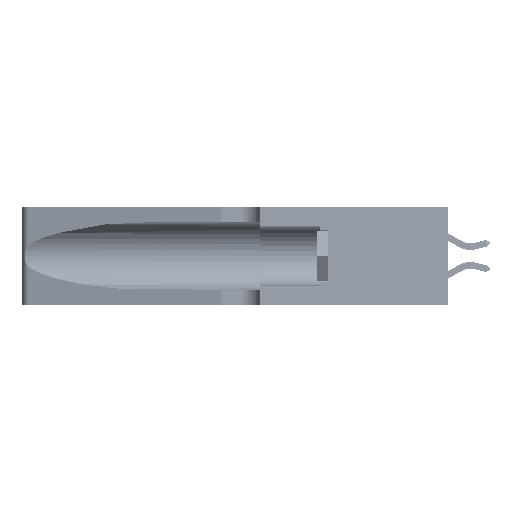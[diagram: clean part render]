
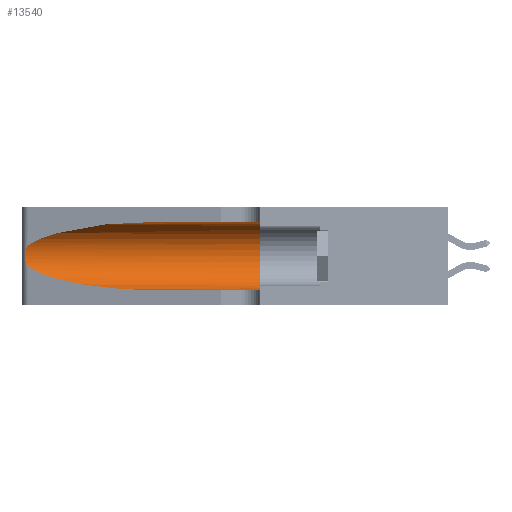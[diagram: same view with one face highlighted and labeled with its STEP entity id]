
A CAD part, left-side view. The second image highlights one B-rep face of the part: STEP entity #13540.
In plain terms, the highlighted cylindrical face has radius 3.308 mm (diameter 6.617 mm), a partial arc.
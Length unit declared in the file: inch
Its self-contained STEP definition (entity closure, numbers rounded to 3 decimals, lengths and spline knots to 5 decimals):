
#231 = CYLINDRICAL_SURFACE ( 'NONE', #7892, 0.13025 ) ;
#562 = VERTEX_POINT ( 'NONE', #39271 ) ;
#3092 = CARTESIAN_POINT ( 'NONE',  ( 0.26075, 1.23896, 0.19203 ) ) ;
#3158 = EDGE_CURVE ( 'NONE', #21313, #7863, #35314, .T. ) ;
#3285 = ORIENTED_EDGE ( 'NONE', *, *, #41470, .F. ) ;
#3637 = CARTESIAN_POINT ( 'NONE',  ( 0.1305, 0.35, 0.185 ) ) ;
#3940 = VERTEX_POINT ( 'NONE', #49144 ) ;
#5099 = EDGE_CURVE ( 'NONE', #7863, #42348, #49323, .T. ) ;
#7113 = CARTESIAN_POINT ( 'NONE',  ( 0.26017, 1.23833, 0.17102 ) ) ;
#7657 = DIRECTION ( 'NONE',  ( 0., 0., 1. ) ) ;
#7863 = VERTEX_POINT ( 'NONE', #19036 ) ;
#7892 = AXIS2_PLACEMENT_3D ( 'NONE', #17090, #48518, #28967 ) ;
#10214 = CARTESIAN_POINT ( 'NONE',  ( 0.18966, 0.96281, 0.31525 ) ) ;
#11119 = CARTESIAN_POINT ( 'NONE',  ( 0.25789, 1.23486, 0.15765 ) ) ;
#11977 = ORIENTED_EDGE ( 'NONE', *, *, #20928, .T. ) ;
#12766 = DIRECTION ( 'NONE',  ( 0., -1., 0. ) ) ;
#13540 = ADVANCED_FACE ( 'NONE', ( #22556 ), #231, .F. ) ;
#14172 = CARTESIAN_POINT ( 'NONE',  ( 0.1305, 0.72297, 0.31525 ) ) ;
#15066 = CARTESIAN_POINT ( 'NONE',  ( 0.25555, 1.22993, 0.14849 ) ) ;
#15588 = CARTESIAN_POINT ( 'NONE',  ( 0.18966, 0.96281, 0.05475 ) ) ;
#17090 = CARTESIAN_POINT ( 'NONE',  ( 0.1305, 1.61858, 0.185 ) ) ;
#18164 = CARTESIAN_POINT ( 'NONE',  ( 0.2373, 1.15595, 0.28018 ) ) ;
#18885 = LINE ( 'NONE', #38609, #38616 ) ;
#18965 = DIRECTION ( 'NONE',  ( 0., -1., 0. ) ) ;
#19036 = CARTESIAN_POINT ( 'NONE',  ( 0.1305, 0.72297, 0.05475 ) ) ;
#19726 = CIRCLE ( 'NONE', #27822, 0.13025 ) ;
#20928 = EDGE_CURVE ( 'NONE', #32905, #562, #31513, .T. ) ;
#21313 = VERTEX_POINT ( 'NONE', #24300 ) ;
#22294 = B_SPLINE_CURVE_WITH_KNOTS ( 'NONE', 3,
 ( #38512, #42462, #46355, #22766, #50283, #26758, #3092, #30759, #7113, #34728, #11119, #38680, #15066, #42628 ),
 .UNSPECIFIED., .F., .F.,
 ( 4, 2, 2, 2, 2, 2, 4 ),
 ( 0., 0.00027, 0.00053, 0.00107, 0.0016, 0.00187, 0.00214 ),
 .UNSPECIFIED. ) ;
#22556 = FACE_OUTER_BOUND ( 'NONE', #27372, .T. ) ;
#22766 = CARTESIAN_POINT ( 'NONE',  ( 0.25787, 1.23484, 0.2124 ) ) ;
#23468 = CARTESIAN_POINT ( 'NONE',  ( 0.25487, 1.22718, 0.14631 ) ) ;
#23604 = EDGE_CURVE ( 'NONE', #562, #21313, #22294, .T. ) ;
#24300 = CARTESIAN_POINT ( 'NONE',  ( 0.25487, 1.22718, 0.14631 ) ) ;
#26758 = CARTESIAN_POINT ( 'NONE',  ( 0.26018, 1.23835, 0.19895 ) ) ;
#27372 = EDGE_LOOP ( 'NONE', ( #11977, #45819, #47043, #49509, #50720, #3285 ) ) ;
#27460 = CARTESIAN_POINT ( 'NONE',  ( 0.1305, 0.72297, 0.05475 ) ) ;
#27822 = AXIS2_PLACEMENT_3D ( 'NONE', #3637, #31306, #7657 ) ;
#28967 = DIRECTION ( 'NONE',  ( 0., 0., -1. ) ) ;
#30759 = CARTESIAN_POINT ( 'NONE',  ( 0.26075, 1.23896, 0.178 ) ) ;
#31306 = DIRECTION ( 'NONE',  ( 0., 1., 0. ) ) ;
#31513 =( BOUNDED_CURVE ( )  B_SPLINE_CURVE ( 3, ( #14172, #10214, #18164, #45656 ),
 .UNSPECIFIED., .F., .F. ) 
 B_SPLINE_CURVE_WITH_KNOTS ( ( 4, 4 ),
 ( 1.5708, 2.84003 ),
 .UNSPECIFIED. ) 
 CURVE ( )  GEOMETRIC_REPRESENTATION_ITEM ( )  RATIONAL_B_SPLINE_CURVE ( ( 1., 0.87, 0.87, 1. ) ) 
 REPRESENTATION_ITEM ( '' )  );
#32905 = VERTEX_POINT ( 'NONE', #49555 ) ;
#34728 = CARTESIAN_POINT ( 'NONE',  ( 0.25856, 1.23593, 0.16098 ) ) ;
#35314 =( BOUNDED_CURVE ( )  B_SPLINE_CURVE ( 3, ( #23468, #39213, #15588, #27460 ),
 .UNSPECIFIED., .F., .F. ) 
 B_SPLINE_CURVE_WITH_KNOTS ( ( 4, 4 ),
 ( 3.44316, 4.71239 ),
 .UNSPECIFIED. ) 
 CURVE ( )  GEOMETRIC_REPRESENTATION_ITEM ( )  RATIONAL_B_SPLINE_CURVE ( ( 1., 0.87, 0.87, 1. ) ) 
 REPRESENTATION_ITEM ( '' )  );
#36386 = CARTESIAN_POINT ( 'NONE',  ( 0.1305, 1.61858, 0.05475 ) ) ;
#38512 = CARTESIAN_POINT ( 'NONE',  ( 0.25487, 1.22718, 0.22369 ) ) ;
#38609 = CARTESIAN_POINT ( 'NONE',  ( 0.1305, 1.61858, 0.31525 ) ) ;
#38616 = VECTOR ( 'NONE', #18965, 39.37008 ) ;
#38680 = CARTESIAN_POINT ( 'NONE',  ( 0.25639, 1.23186, 0.15144 ) ) ;
#39213 = CARTESIAN_POINT ( 'NONE',  ( 0.2373, 1.15595, 0.08982 ) ) ;
#39271 = CARTESIAN_POINT ( 'NONE',  ( 0.25487, 1.22718, 0.22369 ) ) ;
#41470 = EDGE_CURVE ( 'NONE', #32905, #3940, #18885, .T. ) ;
#42202 = EDGE_CURVE ( 'NONE', #3940, #42348, #19726, .T. ) ;
#42348 = VERTEX_POINT ( 'NONE', #43827 ) ;
#42462 = CARTESIAN_POINT ( 'NONE',  ( 0.25555, 1.22994, 0.2215 ) ) ;
#42628 = CARTESIAN_POINT ( 'NONE',  ( 0.25487, 1.22718, 0.14631 ) ) ;
#43827 = CARTESIAN_POINT ( 'NONE',  ( 0.1305, 0.35, 0.05475 ) ) ;
#45656 = CARTESIAN_POINT ( 'NONE',  ( 0.25487, 1.22718, 0.22369 ) ) ;
#45819 = ORIENTED_EDGE ( 'NONE', *, *, #23604, .T. ) ;
#46355 = CARTESIAN_POINT ( 'NONE',  ( 0.25639, 1.23184, 0.21858 ) ) ;
#47043 = ORIENTED_EDGE ( 'NONE', *, *, #3158, .T. ) ;
#48113 = VECTOR ( 'NONE', #12766, 39.37008 ) ;
#48518 = DIRECTION ( 'NONE',  ( 0., -1., 0. ) ) ;
#49144 = CARTESIAN_POINT ( 'NONE',  ( 0.1305, 0.35, 0.31525 ) ) ;
#49323 = LINE ( 'NONE', #36386, #48113 ) ;
#49509 = ORIENTED_EDGE ( 'NONE', *, *, #5099, .T. ) ;
#49555 = CARTESIAN_POINT ( 'NONE',  ( 0.1305, 0.72297, 0.31525 ) ) ;
#50283 = CARTESIAN_POINT ( 'NONE',  ( 0.25854, 1.2359, 0.20912 ) ) ;
#50720 = ORIENTED_EDGE ( 'NONE', *, *, #42202, .F. ) ;
